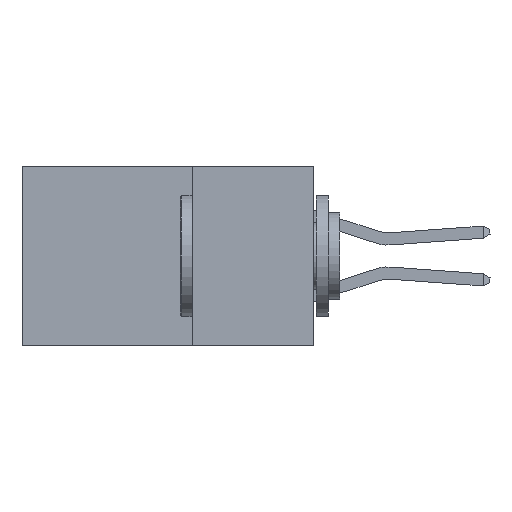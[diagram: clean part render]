
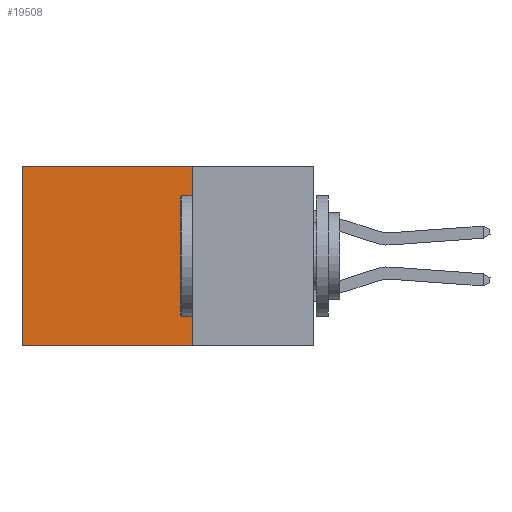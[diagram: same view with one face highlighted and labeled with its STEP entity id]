
A CAD part, left-side view. The second image highlights one B-rep face of the part: STEP entity #19508.
In plain terms, the highlighted planar face has unit normal (-1, 0, 0).
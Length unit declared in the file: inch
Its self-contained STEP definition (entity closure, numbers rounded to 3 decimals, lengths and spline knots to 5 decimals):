
#350 = CARTESIAN_POINT ( 'NONE',  ( 0.2875, 0.25, 0. ) ) ;
#844 = CARTESIAN_POINT ( 'NONE',  ( 0.2875, 0.25, 0. ) ) ;
#2184 = CARTESIAN_POINT ( 'NONE',  ( 0.2875, 0.6, -0.37 ) ) ;
#3022 = EDGE_CURVE ( 'NONE', #20965, #20074, #39344, .T. ) ;
#3671 = ORIENTED_EDGE ( 'NONE', *, *, #3022, .T. ) ;
#4321 = VECTOR ( 'NONE', #43653, 39.37008 ) ;
#5994 = DIRECTION ( 'NONE',  ( 0., 0., -1. ) ) ;
#7524 = DIRECTION ( 'NONE',  ( 0., 0., -1. ) ) ;
#9043 = EDGE_LOOP ( 'NONE', ( #3671, #41420, #29616, #41978 ) ) ;
#9567 = CARTESIAN_POINT ( 'NONE',  ( 0.2875, 0.25, 0. ) ) ;
#10437 = LINE ( 'NONE', #21295, #34941 ) ;
#14724 = CARTESIAN_POINT ( 'NONE',  ( 0.2875, 0.6, 0. ) ) ;
#15617 = CARTESIAN_POINT ( 'NONE',  ( 0.2875, 0.25, -0.37 ) ) ;
#17191 = FACE_OUTER_BOUND ( 'NONE', #9043, .T. ) ;
#17819 = DIRECTION ( 'NONE',  ( 0., 0., -1. ) ) ;
#19508 = ADVANCED_FACE ( 'NONE', ( #17191 ), #41179, .F. ) ;
#20074 = VERTEX_POINT ( 'NONE', #2184 ) ;
#20635 = DIRECTION ( 'NONE',  ( 1., 0., 0. ) ) ;
#20965 = VERTEX_POINT ( 'NONE', #38191 ) ;
#21295 = CARTESIAN_POINT ( 'NONE',  ( 0.2875, 0.25, -0.37 ) ) ;
#22586 = AXIS2_PLACEMENT_3D ( 'NONE', #350, #20635, #17819 ) ;
#26782 = VERTEX_POINT ( 'NONE', #15617 ) ;
#29616 = ORIENTED_EDGE ( 'NONE', *, *, #43702, .F. ) ;
#30279 = VECTOR ( 'NONE', #7524, 39.37008 ) ;
#30562 = EDGE_CURVE ( 'NONE', #26782, #20074, #10437, .T. ) ;
#31520 = LINE ( 'NONE', #9567, #4321 ) ;
#33176 = VECTOR ( 'NONE', #5994, 39.37008 ) ;
#33390 = CARTESIAN_POINT ( 'NONE',  ( 0.2875, 0.25, 0. ) ) ;
#34941 = VECTOR ( 'NONE', #35116, 39.37008 ) ;
#35116 = DIRECTION ( 'NONE',  ( 0., 1., 0. ) ) ;
#38191 = CARTESIAN_POINT ( 'NONE',  ( 0.2875, 0.6, 0. ) ) ;
#38335 = VERTEX_POINT ( 'NONE', #844 ) ;
#38648 = EDGE_CURVE ( 'NONE', #38335, #20965, #31520, .T. ) ;
#39344 = LINE ( 'NONE', #14724, #30279 ) ;
#39604 = LINE ( 'NONE', #33390, #33176 ) ;
#41179 = PLANE ( 'NONE',  #22586 ) ;
#41420 = ORIENTED_EDGE ( 'NONE', *, *, #30562, .F. ) ;
#41978 = ORIENTED_EDGE ( 'NONE', *, *, #38648, .T. ) ;
#43653 = DIRECTION ( 'NONE',  ( 0., 1., 0. ) ) ;
#43702 = EDGE_CURVE ( 'NONE', #38335, #26782, #39604, .T. ) ;
